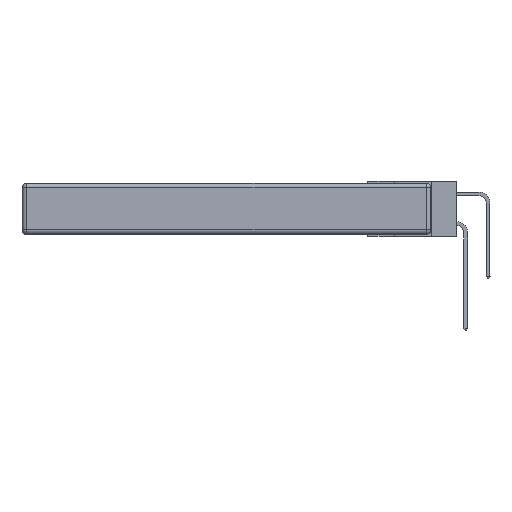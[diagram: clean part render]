
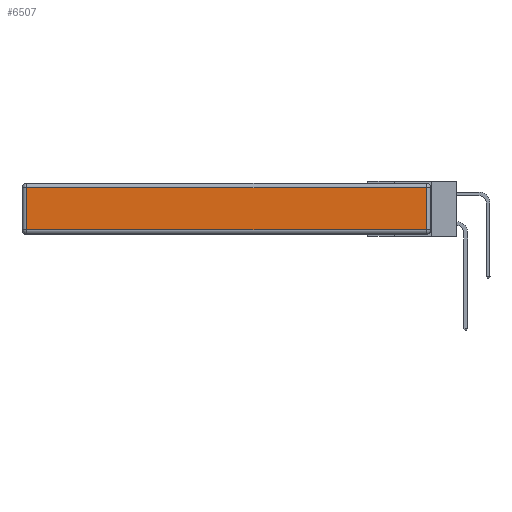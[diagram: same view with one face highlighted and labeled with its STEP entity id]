
A CAD part, left-side view. The second image highlights one B-rep face of the part: STEP entity #6507.
In plain terms, the highlighted planar face has unit normal (-1, 0, 0).
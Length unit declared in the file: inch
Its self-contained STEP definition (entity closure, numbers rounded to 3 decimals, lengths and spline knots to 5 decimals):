
#510 = DIRECTION ( 'NONE',  ( 0., 0., 1. ) ) ;
#1679 = VECTOR ( 'NONE', #12648, 39.37008 ) ;
#3010 = CARTESIAN_POINT ( 'NONE',  ( 0., 2.72, -0.343 ) ) ;
#3265 = CARTESIAN_POINT ( 'NONE',  ( 0., 0., -0.343 ) ) ;
#3289 = DIRECTION ( 'NONE',  ( 0., 1., 0. ) ) ;
#3343 = ORIENTED_EDGE ( 'NONE', *, *, #13427, .T. ) ;
#4065 = EDGE_LOOP ( 'NONE', ( #10975, #3343, #4296, #4520 ) ) ;
#4244 = AXIS2_PLACEMENT_3D ( 'NONE', #3265, #4404, #510 ) ;
#4296 = ORIENTED_EDGE ( 'NONE', *, *, #13414, .T. ) ;
#4404 = DIRECTION ( 'NONE',  ( -1., 0., 0. ) ) ;
#4520 = ORIENTED_EDGE ( 'NONE', *, *, #5930, .T. ) ;
#4739 = VERTEX_POINT ( 'NONE', #5548 ) ;
#5548 = CARTESIAN_POINT ( 'NONE',  ( 0., 0.03, -0.03 ) ) ;
#5835 = DIRECTION ( 'NONE',  ( 0., 0., 1. ) ) ;
#5930 = EDGE_CURVE ( 'NONE', #15680, #15999, #12694, .T. ) ;
#6143 = VERTEX_POINT ( 'NONE', #9003 ) ;
#6507 = ADVANCED_FACE ( 'NONE', ( #10086 ), #11443, .T. ) ;
#6611 = EDGE_CURVE ( 'NONE', #15999, #6143, #15456, .T. ) ;
#7161 = CARTESIAN_POINT ( 'NONE',  ( 0., 0.03, -0.343 ) ) ;
#9003 = CARTESIAN_POINT ( 'NONE',  ( 0., 0.03, -0.313 ) ) ;
#9617 = DIRECTION ( 'NONE',  ( 0., -1., 0. ) ) ;
#10086 = FACE_OUTER_BOUND ( 'NONE', #4065, .T. ) ;
#10794 = VECTOR ( 'NONE', #5835, 39.37008 ) ;
#10825 = CARTESIAN_POINT ( 'NONE',  ( 0., 0., -0.313 ) ) ;
#10975 = ORIENTED_EDGE ( 'NONE', *, *, #6611, .T. ) ;
#11223 = LINE ( 'NONE', #7161, #10794 ) ;
#11443 = PLANE ( 'NONE',  #4244 ) ;
#12648 = DIRECTION ( 'NONE',  ( 0., 0., -1. ) ) ;
#12694 = LINE ( 'NONE', #3010, #1679 ) ;
#13414 = EDGE_CURVE ( 'NONE', #4739, #15680, #14896, .T. ) ;
#13427 = EDGE_CURVE ( 'NONE', #6143, #4739, #11223, .T. ) ;
#14558 = CARTESIAN_POINT ( 'NONE',  ( 0., 2.72, -0.03 ) ) ;
#14592 = VECTOR ( 'NONE', #9617, 39.37008 ) ;
#14896 = LINE ( 'NONE', #15580, #16181 ) ;
#15456 = LINE ( 'NONE', #10825, #14592 ) ;
#15580 = CARTESIAN_POINT ( 'NONE',  ( 0., 2.75, -0.03 ) ) ;
#15680 = VERTEX_POINT ( 'NONE', #14558 ) ;
#15999 = VERTEX_POINT ( 'NONE', #17848 ) ;
#16181 = VECTOR ( 'NONE', #3289, 39.37008 ) ;
#17848 = CARTESIAN_POINT ( 'NONE',  ( 0., 2.72, -0.313 ) ) ;
